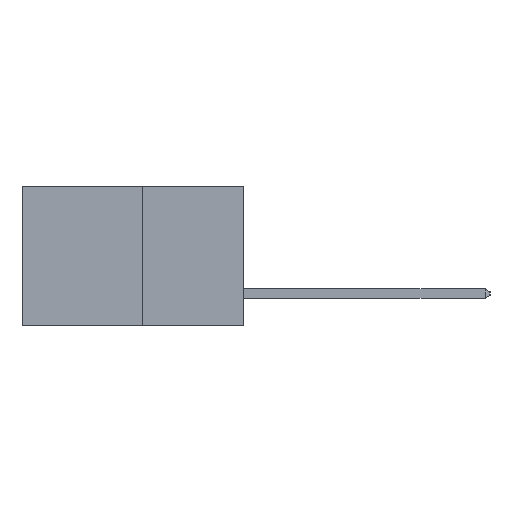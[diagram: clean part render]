
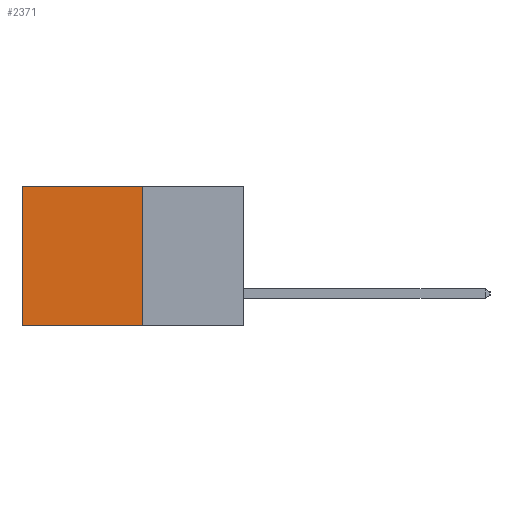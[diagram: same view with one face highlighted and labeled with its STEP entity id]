
A CAD part, left-side view. The second image highlights one B-rep face of the part: STEP entity #2371.
In plain terms, the highlighted planar face has unit normal (-1, 0, 0).
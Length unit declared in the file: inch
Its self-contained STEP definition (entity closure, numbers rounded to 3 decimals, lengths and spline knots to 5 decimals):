
#368 = VERTEX_POINT ( 'NONE', #6991 ) ;
#594 = CARTESIAN_POINT ( 'NONE',  ( 0.277, 0.27, 0. ) ) ;
#747 = VECTOR ( 'NONE', #4345, 39.37008 ) ;
#901 = EDGE_CURVE ( 'NONE', #1336, #2505, #1770, .T. ) ;
#1336 = VERTEX_POINT ( 'NONE', #594 ) ;
#1518 = EDGE_CURVE ( 'NONE', #1336, #368, #7372, .T. ) ;
#1733 = FACE_OUTER_BOUND ( 'NONE', #7404, .T. ) ;
#1768 = CARTESIAN_POINT ( 'NONE',  ( 0.277, 0.27, -0.37 ) ) ;
#1770 = LINE ( 'NONE', #1768, #8178 ) ;
#1897 = ORIENTED_EDGE ( 'NONE', *, *, #6041, .T. ) ;
#2371 = ADVANCED_FACE ( 'NONE', ( #1733 ), #6951, .F. ) ;
#2462 = CARTESIAN_POINT ( 'NONE',  ( 0.277, 0.27, -0.37 ) ) ;
#2505 = VERTEX_POINT ( 'NONE', #2462 ) ;
#2592 = VECTOR ( 'NONE', #5859, 39.37008 ) ;
#3434 = ORIENTED_EDGE ( 'NONE', *, *, #1518, .T. ) ;
#3449 = ORIENTED_EDGE ( 'NONE', *, *, #7075, .F. ) ;
#3462 = ORIENTED_EDGE ( 'NONE', *, *, #901, .F. ) ;
#4306 = LINE ( 'NONE', #6051, #2592 ) ;
#4323 = VECTOR ( 'NONE', #4996, 39.37008 ) ;
#4345 = DIRECTION ( 'NONE',  ( 0., 1., 0. ) ) ;
#4987 = AXIS2_PLACEMENT_3D ( 'NONE', #7599, #6721, #7055 ) ;
#4996 = DIRECTION ( 'NONE',  ( 0., 1., 0. ) ) ;
#5036 = CARTESIAN_POINT ( 'NONE',  ( 0.277, 0.27, -0.37 ) ) ;
#5591 = VERTEX_POINT ( 'NONE', #6854 ) ;
#5859 = DIRECTION ( 'NONE',  ( 0., 0., -1. ) ) ;
#6041 = EDGE_CURVE ( 'NONE', #368, #5591, #4306, .T. ) ;
#6051 = CARTESIAN_POINT ( 'NONE',  ( 0.277, 0.59, -0.37 ) ) ;
#6721 = DIRECTION ( 'NONE',  ( 1., 0., 0. ) ) ;
#6722 = CARTESIAN_POINT ( 'NONE',  ( 0.277, 0.27, 0. ) ) ;
#6854 = CARTESIAN_POINT ( 'NONE',  ( 0.277, 0.59, -0.37 ) ) ;
#6951 = PLANE ( 'NONE',  #4987 ) ;
#6991 = CARTESIAN_POINT ( 'NONE',  ( 0.277, 0.59, 0. ) ) ;
#7055 = DIRECTION ( 'NONE',  ( 0., 0., -1. ) ) ;
#7075 = EDGE_CURVE ( 'NONE', #2505, #5591, #7517, .T. ) ;
#7372 = LINE ( 'NONE', #6722, #747 ) ;
#7404 = EDGE_LOOP ( 'NONE', ( #1897, #3449, #3462, #3434 ) ) ;
#7517 = LINE ( 'NONE', #5036, #4323 ) ;
#7599 = CARTESIAN_POINT ( 'NONE',  ( 0.277, 0.27, -0.37 ) ) ;
#8178 = VECTOR ( 'NONE', #8213, 39.37008 ) ;
#8213 = DIRECTION ( 'NONE',  ( 0., 0., -1. ) ) ;
